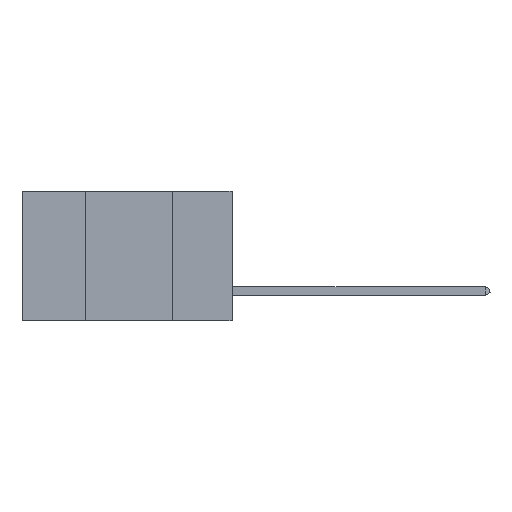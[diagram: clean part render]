
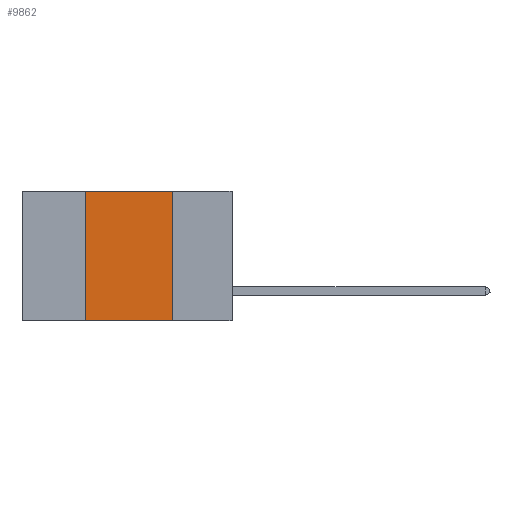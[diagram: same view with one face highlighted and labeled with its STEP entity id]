
A CAD part, left-side view. The second image highlights one B-rep face of the part: STEP entity #9862.
In plain terms, the highlighted planar face has unit normal (-1, 0, 0).
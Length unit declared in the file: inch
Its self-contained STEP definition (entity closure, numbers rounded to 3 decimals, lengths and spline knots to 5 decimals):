
#495 = CARTESIAN_POINT ( 'NONE',  ( 0., 0.17, 0. ) ) ;
#542 = ORIENTED_EDGE ( 'NONE', *, *, #20691, .F. ) ;
#1704 = VERTEX_POINT ( 'NONE', #495 ) ;
#1722 = VECTOR ( 'NONE', #5043, 39.37008 ) ;
#1752 = VERTEX_POINT ( 'NONE', #17667 ) ;
#2627 = DIRECTION ( 'NONE',  ( 1., 0., 0. ) ) ;
#2689 = CARTESIAN_POINT ( 'NONE',  ( 0., 0.6, -0.37 ) ) ;
#2709 = ORIENTED_EDGE ( 'NONE', *, *, #16326, .T. ) ;
#2960 = VECTOR ( 'NONE', #7497, 39.37008 ) ;
#3002 = LINE ( 'NONE', #6895, #5412 ) ;
#4835 = LINE ( 'NONE', #2689, #2960 ) ;
#5043 = DIRECTION ( 'NONE',  ( 0., -1., 0. ) ) ;
#5412 = VECTOR ( 'NONE', #17581, 39.37008 ) ;
#6087 = CARTESIAN_POINT ( 'NONE',  ( 0., 0.17, -0.37 ) ) ;
#6426 = CARTESIAN_POINT ( 'NONE',  ( 0., 0.6, 0. ) ) ;
#6895 = CARTESIAN_POINT ( 'NONE',  ( 0., 0.17, 0. ) ) ;
#7497 = DIRECTION ( 'NONE',  ( 0., -1., 0. ) ) ;
#8742 = ORIENTED_EDGE ( 'NONE', *, *, #13723, .F. ) ;
#9230 = ORIENTED_EDGE ( 'NONE', *, *, #10277, .F. ) ;
#9534 = VERTEX_POINT ( 'NONE', #6087 ) ;
#9862 = ADVANCED_FACE ( 'NONE', ( #13080 ), #13030, .F. ) ;
#10277 = EDGE_CURVE ( 'NONE', #1704, #9534, #3002, .T. ) ;
#11386 = CARTESIAN_POINT ( 'NONE',  ( 0., 0.42, 0. ) ) ;
#12470 = VERTEX_POINT ( 'NONE', #17872 ) ;
#13030 = PLANE ( 'NONE',  #16629 ) ;
#13080 = FACE_OUTER_BOUND ( 'NONE', #16681, .T. ) ;
#13723 = EDGE_CURVE ( 'NONE', #12470, #1704, #18186, .T. ) ;
#16326 = EDGE_CURVE ( 'NONE', #1752, #9534, #4835, .T. ) ;
#16473 = CARTESIAN_POINT ( 'NONE',  ( 0., 0.6, 0. ) ) ;
#16629 = AXIS2_PLACEMENT_3D ( 'NONE', #16473, #2627, #20000 ) ;
#16681 = EDGE_LOOP ( 'NONE', ( #9230, #8742, #542, #2709 ) ) ;
#17581 = DIRECTION ( 'NONE',  ( 0., 0., -1. ) ) ;
#17667 = CARTESIAN_POINT ( 'NONE',  ( 0., 0.42, -0.37 ) ) ;
#17872 = CARTESIAN_POINT ( 'NONE',  ( 0., 0.42, 0. ) ) ;
#17998 = VECTOR ( 'NONE', #22150, 39.37008 ) ;
#18186 = LINE ( 'NONE', #6426, #1722 ) ;
#19029 = LINE ( 'NONE', #11386, #17998 ) ;
#20000 = DIRECTION ( 'NONE',  ( 0., 0., -1. ) ) ;
#20691 = EDGE_CURVE ( 'NONE', #1752, #12470, #19029, .T. ) ;
#22150 = DIRECTION ( 'NONE',  ( 0., 0., 1. ) ) ;
